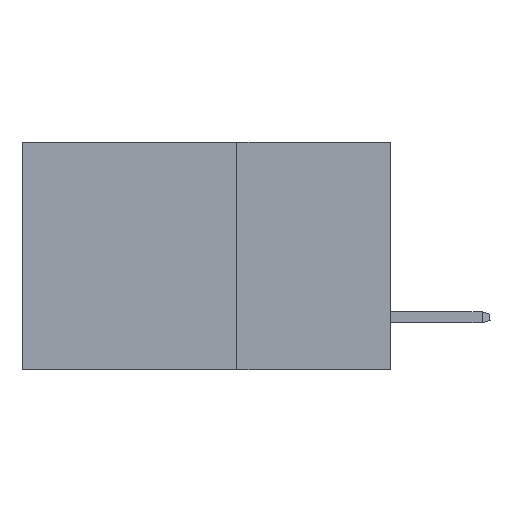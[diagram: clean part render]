
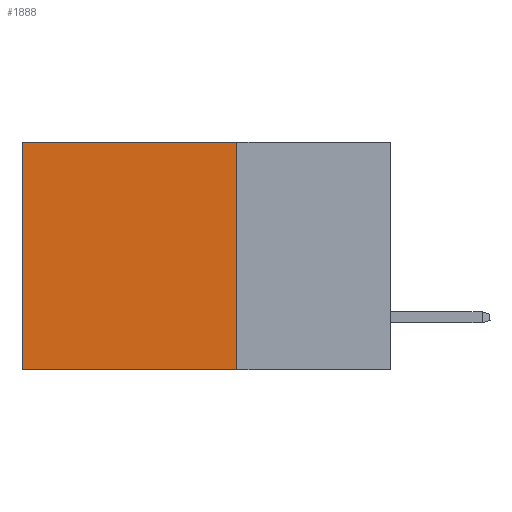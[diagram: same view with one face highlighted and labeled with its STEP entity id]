
A CAD part, left-side view. The second image highlights one B-rep face of the part: STEP entity #1888.
In plain terms, the highlighted planar face has unit normal (-1, 0, 0).
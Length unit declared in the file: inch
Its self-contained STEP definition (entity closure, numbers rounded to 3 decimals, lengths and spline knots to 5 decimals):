
#455 = AXIS2_PLACEMENT_3D ( 'NONE', #5007, #3144, #3182 ) ;
#1034 = CARTESIAN_POINT ( 'NONE',  ( 0.2875, 0.6, 0. ) ) ;
#1888 = ADVANCED_FACE ( 'NONE', ( #14214 ), #11663, .F. ) ;
#2781 = EDGE_CURVE ( 'NONE', #5648, #7500, #7068, .T. ) ;
#2992 = CARTESIAN_POINT ( 'NONE',  ( 0.2875, 0.25, 0. ) ) ;
#3144 = DIRECTION ( 'NONE',  ( 1., 0., 0. ) ) ;
#3182 = DIRECTION ( 'NONE',  ( 0., 0., -1. ) ) ;
#4611 = ORIENTED_EDGE ( 'NONE', *, *, #10588, .T. ) ;
#4626 = ORIENTED_EDGE ( 'NONE', *, *, #11528, .F. ) ;
#5007 = CARTESIAN_POINT ( 'NONE',  ( 0.2875, 0.25, 0. ) ) ;
#5474 = CARTESIAN_POINT ( 'NONE',  ( 0.2875, 0.6, 0. ) ) ;
#5519 = VERTEX_POINT ( 'NONE', #14200 ) ;
#5648 = VERTEX_POINT ( 'NONE', #5474 ) ;
#6399 = DIRECTION ( 'NONE',  ( 0., 0., -1. ) ) ;
#6834 = DIRECTION ( 'NONE',  ( 0., 1., 0. ) ) ;
#7051 = CARTESIAN_POINT ( 'NONE',  ( 0.2875, 0.6, -0.37 ) ) ;
#7068 = LINE ( 'NONE', #1034, #12141 ) ;
#7500 = VERTEX_POINT ( 'NONE', #7051 ) ;
#8154 = ORIENTED_EDGE ( 'NONE', *, *, #2781, .T. ) ;
#8227 = ORIENTED_EDGE ( 'NONE', *, *, #10925, .F. ) ;
#8770 = DIRECTION ( 'NONE',  ( 0., 0., -1. ) ) ;
#9671 = VECTOR ( 'NONE', #6834, 39.37008 ) ;
#9850 = VECTOR ( 'NONE', #12996, 39.37008 ) ;
#10376 = LINE ( 'NONE', #13391, #9671 ) ;
#10588 = EDGE_CURVE ( 'NONE', #5519, #5648, #10376, .T. ) ;
#10925 = EDGE_CURVE ( 'NONE', #13233, #7500, #12640, .T. ) ;
#11397 = LINE ( 'NONE', #2992, #14359 ) ;
#11485 = EDGE_LOOP ( 'NONE', ( #8154, #8227, #4626, #4611 ) ) ;
#11528 = EDGE_CURVE ( 'NONE', #5519, #13233, #11397, .T. ) ;
#11663 = PLANE ( 'NONE',  #455 ) ;
#12141 = VECTOR ( 'NONE', #8770, 39.37008 ) ;
#12640 = LINE ( 'NONE', #14013, #9850 ) ;
#12996 = DIRECTION ( 'NONE',  ( 0., 1., 0. ) ) ;
#13138 = CARTESIAN_POINT ( 'NONE',  ( 0.2875, 0.25, -0.37 ) ) ;
#13233 = VERTEX_POINT ( 'NONE', #13138 ) ;
#13391 = CARTESIAN_POINT ( 'NONE',  ( 0.2875, 0.25, 0. ) ) ;
#14013 = CARTESIAN_POINT ( 'NONE',  ( 0.2875, 0.25, -0.37 ) ) ;
#14200 = CARTESIAN_POINT ( 'NONE',  ( 0.2875, 0.25, 0. ) ) ;
#14214 = FACE_OUTER_BOUND ( 'NONE', #11485, .T. ) ;
#14359 = VECTOR ( 'NONE', #6399, 39.37008 ) ;
